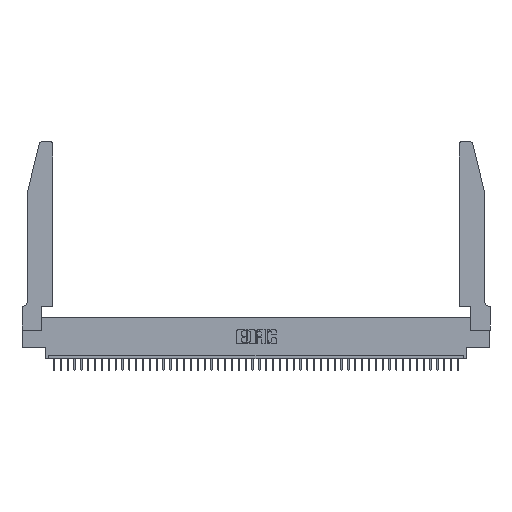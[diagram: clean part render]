
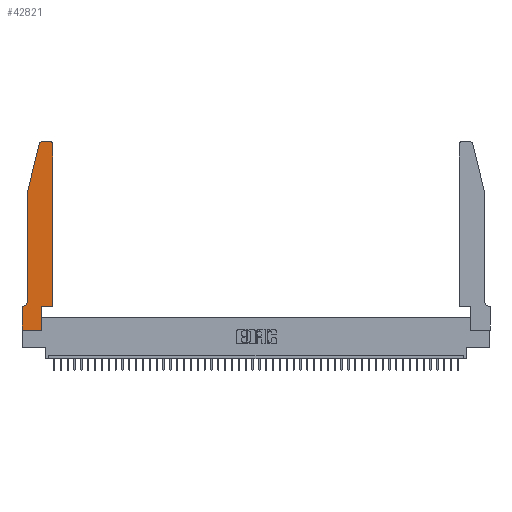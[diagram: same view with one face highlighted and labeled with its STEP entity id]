
A CAD part, top view. The second image highlights one B-rep face of the part: STEP entity #42821.
In plain terms, the highlighted planar face has unit normal (0, 0, 1).
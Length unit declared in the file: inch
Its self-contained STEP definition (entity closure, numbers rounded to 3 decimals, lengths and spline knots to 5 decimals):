
#1386 = EDGE_CURVE ( 'NONE', #28269, #39995, #18766, .T. ) ;
#1595 = DIRECTION ( 'NONE',  ( 0., -1., 0. ) ) ;
#1728 = CARTESIAN_POINT ( 'NONE',  ( 0.0755, 2., 0.37 ) ) ;
#1734 = EDGE_CURVE ( 'NONE', #41460, #28269, #22778, .T. ) ;
#1901 = EDGE_CURVE ( 'NONE', #10753, #26854, #19281, .T. ) ;
#2366 = CARTESIAN_POINT ( 'NONE',  ( 0.4505, 2.72, 0.37 ) ) ;
#2916 = ORIENTED_EDGE ( 'NONE', *, *, #42637, .T. ) ;
#3368 = PLANE ( 'NONE',  #34257 ) ;
#4056 = DIRECTION ( 'NONE',  ( 0., 1., 0. ) ) ;
#4439 = ORIENTED_EDGE ( 'NONE', *, *, #39671, .T. ) ;
#5008 = EDGE_CURVE ( 'NONE', #9063, #17050, #12805, .T. ) ;
#5109 = VERTEX_POINT ( 'NONE', #29604 ) ;
#5264 = CARTESIAN_POINT ( 'NONE',  ( 0.25487, 2.72718, 0.37 ) ) ;
#5445 = LINE ( 'NONE', #16373, #17559 ) ;
#5502 = EDGE_CURVE ( 'NONE', #26854, #41460, #25385, .T. ) ;
#5588 = VECTOR ( 'NONE', #44332, 39.37008 ) ;
#5846 = ORIENTED_EDGE ( 'NONE', *, *, #1901, .T. ) ;
#6260 = ORIENTED_EDGE ( 'NONE', *, *, #43739, .T. ) ;
#7249 = DIRECTION ( 'NONE',  ( 1., 0., 0. ) ) ;
#7957 = EDGE_LOOP ( 'NONE', ( #5846, #20484, #26499, #13925, #24189, #12113, #4439, #11644, #6260, #42719, #10710, #2916 ) ) ;
#8633 = LINE ( 'NONE', #20446, #16722 ) ;
#8942 = DIRECTION ( 'NONE',  ( -1., 0., 0. ) ) ;
#9063 = VERTEX_POINT ( 'NONE', #15817 ) ;
#9669 = CARTESIAN_POINT ( 'NONE',  ( 0.2865, 0., 0.37 ) ) ;
#9726 = FACE_OUTER_BOUND ( 'NONE', #7957, .T. ) ;
#10149 = EDGE_CURVE ( 'NONE', #44772, #21657, #5445, .T. ) ;
#10412 = DIRECTION ( 'NONE',  ( 1., 0., 0. ) ) ;
#10710 = ORIENTED_EDGE ( 'NONE', *, *, #10149, .T. ) ;
#10753 = VERTEX_POINT ( 'NONE', #34046 ) ;
#11279 = VECTOR ( 'NONE', #18706, 39.37008 ) ;
#11644 = ORIENTED_EDGE ( 'NONE', *, *, #42261, .T. ) ;
#12113 = ORIENTED_EDGE ( 'NONE', *, *, #5008, .T. ) ;
#12209 = CIRCLE ( 'NONE', #28070, 0.07 ) ;
#12227 = CARTESIAN_POINT ( 'NONE',  ( 0., 0., 0.37 ) ) ;
#12381 = AXIS2_PLACEMENT_3D ( 'NONE', #17077, #35890, #24946 ) ;
#12805 = LINE ( 'NONE', #43579, #28364 ) ;
#13925 = ORIENTED_EDGE ( 'NONE', *, *, #1386, .T. ) ;
#14214 = VERTEX_POINT ( 'NONE', #9669 ) ;
#15817 = CARTESIAN_POINT ( 'NONE',  ( 0.0055, 0.35, 0.37 ) ) ;
#16373 = CARTESIAN_POINT ( 'NONE',  ( 0.4505, 0.35, 0.37 ) ) ;
#16722 = VECTOR ( 'NONE', #24150, 39.37008 ) ;
#17050 = VERTEX_POINT ( 'NONE', #46565 ) ;
#17077 = CARTESIAN_POINT ( 'NONE',  ( 0.4205, 2.72, 0.37 ) ) ;
#17559 = VECTOR ( 'NONE', #24393, 39.37008 ) ;
#17855 = LINE ( 'NONE', #28867, #33891 ) ;
#17862 = CARTESIAN_POINT ( 'NONE',  ( 0.0755, 0.42, 0.37 ) ) ;
#18263 = DIRECTION ( 'NONE',  ( 0., 0., -1. ) ) ;
#18611 = CARTESIAN_POINT ( 'NONE',  ( 0.0755, 2., 0.37 ) ) ;
#18706 = DIRECTION ( 'NONE',  ( -0.239, -0.971, 0. ) ) ;
#18766 = LINE ( 'NONE', #18611, #5588 ) ;
#18959 = EDGE_CURVE ( 'NONE', #39995, #9063, #12209, .T. ) ;
#19281 = LINE ( 'NONE', #30285, #47015 ) ;
#20262 = EDGE_CURVE ( 'NONE', #5109, #44772, #8633, .T. ) ;
#20446 = CARTESIAN_POINT ( 'NONE',  ( 0.4505, 0.35, 0.37 ) ) ;
#20484 = ORIENTED_EDGE ( 'NONE', *, *, #5502, .T. ) ;
#21657 = VERTEX_POINT ( 'NONE', #2366 ) ;
#21701 = DIRECTION ( 'NONE',  ( 0., 0., 1. ) ) ;
#22778 = LINE ( 'NONE', #1728, #11279 ) ;
#23480 = LINE ( 'NONE', #37519, #40736 ) ;
#24150 = DIRECTION ( 'NONE',  ( 1., 0., 0. ) ) ;
#24189 = ORIENTED_EDGE ( 'NONE', *, *, #18959, .T. ) ;
#24393 = DIRECTION ( 'NONE',  ( 0., 1., 0. ) ) ;
#24946 = DIRECTION ( 'NONE',  ( 1., 0., 0. ) ) ;
#25079 = DIRECTION ( 'NONE',  ( -1., 0., 0. ) ) ;
#25385 = CIRCLE ( 'NONE', #27876, 0.03 ) ;
#26499 = ORIENTED_EDGE ( 'NONE', *, *, #1734, .T. ) ;
#26854 = VERTEX_POINT ( 'NONE', #46907 ) ;
#27876 = AXIS2_PLACEMENT_3D ( 'NONE', #36568, #32439, #10412 ) ;
#28070 = AXIS2_PLACEMENT_3D ( 'NONE', #40296, #18263, #47559 ) ;
#28269 = VERTEX_POINT ( 'NONE', #41281 ) ;
#28364 = VECTOR ( 'NONE', #25079, 39.37008 ) ;
#28867 = CARTESIAN_POINT ( 'NONE',  ( 0., 0., 0.37 ) ) ;
#29270 = CARTESIAN_POINT ( 'NONE',  ( 0., 0.35, 0.37 ) ) ;
#29604 = CARTESIAN_POINT ( 'NONE',  ( 0.2865, 0.35, 0.37 ) ) ;
#29875 = VERTEX_POINT ( 'NONE', #31578 ) ;
#30285 = CARTESIAN_POINT ( 'NONE',  ( 0.2605, 2.75, 0.37 ) ) ;
#31295 = CARTESIAN_POINT ( 'NONE',  ( 0.4505, 0.35, 0.37 ) ) ;
#31578 = CARTESIAN_POINT ( 'NONE',  ( 0., 0., 0.37 ) ) ;
#32439 = DIRECTION ( 'NONE',  ( 0., 0., 1. ) ) ;
#33891 = VECTOR ( 'NONE', #47064, 39.37008 ) ;
#34046 = CARTESIAN_POINT ( 'NONE',  ( 0.4205, 2.75, 0.37 ) ) ;
#34257 = AXIS2_PLACEMENT_3D ( 'NONE', #29270, #21701, #7249 ) ;
#35890 = DIRECTION ( 'NONE',  ( 0., 0., 1. ) ) ;
#36568 = CARTESIAN_POINT ( 'NONE',  ( 0.284, 2.72, 0.37 ) ) ;
#36690 = VECTOR ( 'NONE', #1595, 39.37008 ) ;
#37519 = CARTESIAN_POINT ( 'NONE',  ( 0.2865, 0.35, 0.37 ) ) ;
#39671 = EDGE_CURVE ( 'NONE', #17050, #29875, #46549, .T. ) ;
#39995 = VERTEX_POINT ( 'NONE', #17862 ) ;
#40296 = CARTESIAN_POINT ( 'NONE',  ( 0.0055, 0.42, 0.37 ) ) ;
#40736 = VECTOR ( 'NONE', #4056, 39.37008 ) ;
#41281 = CARTESIAN_POINT ( 'NONE',  ( 0.0755, 2., 0.37 ) ) ;
#41460 = VERTEX_POINT ( 'NONE', #5264 ) ;
#42261 = EDGE_CURVE ( 'NONE', #29875, #14214, #17855, .T. ) ;
#42637 = EDGE_CURVE ( 'NONE', #21657, #10753, #47703, .T. ) ;
#42719 = ORIENTED_EDGE ( 'NONE', *, *, #20262, .T. ) ;
#42821 = ADVANCED_FACE ( 'NONE', ( #9726 ), #3368, .T. ) ;
#43579 = CARTESIAN_POINT ( 'NONE',  ( 0.0755, 0.35, 0.37 ) ) ;
#43739 = EDGE_CURVE ( 'NONE', #14214, #5109, #23480, .T. ) ;
#44332 = DIRECTION ( 'NONE',  ( 0., -1., 0. ) ) ;
#44772 = VERTEX_POINT ( 'NONE', #31295 ) ;
#46549 = LINE ( 'NONE', #12227, #36690 ) ;
#46565 = CARTESIAN_POINT ( 'NONE',  ( 0., 0.35, 0.37 ) ) ;
#46907 = CARTESIAN_POINT ( 'NONE',  ( 0.284, 2.75, 0.37 ) ) ;
#47015 = VECTOR ( 'NONE', #8942, 39.37008 ) ;
#47064 = DIRECTION ( 'NONE',  ( 1., 0., 0. ) ) ;
#47559 = DIRECTION ( 'NONE',  ( -1., 0., 0. ) ) ;
#47703 = CIRCLE ( 'NONE', #12381, 0.03 ) ;
